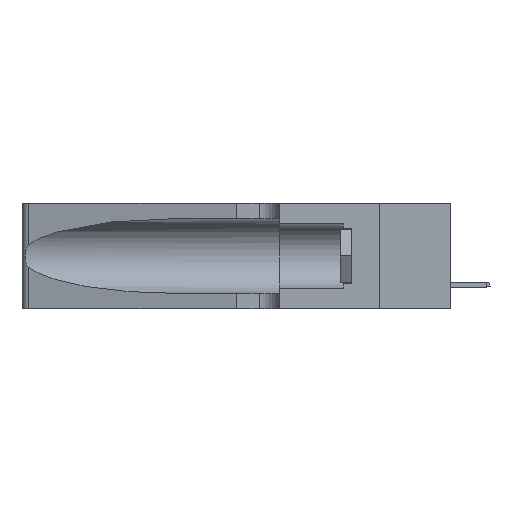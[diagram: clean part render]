
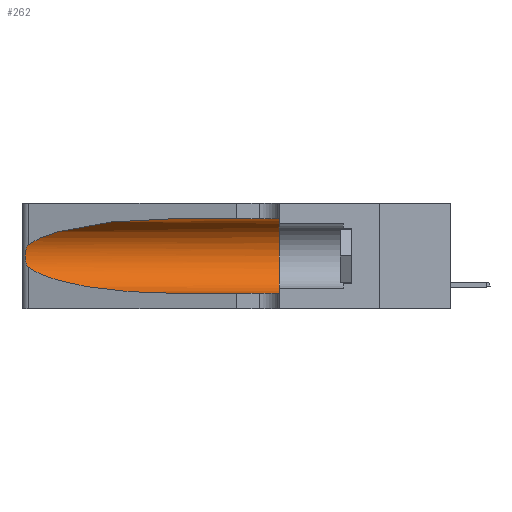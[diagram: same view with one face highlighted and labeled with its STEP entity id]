
A CAD part, left-side view. The second image highlights one B-rep face of the part: STEP entity #262.
In plain terms, the highlighted cylindrical face has radius 3.308 mm (diameter 6.617 mm), a partial arc.
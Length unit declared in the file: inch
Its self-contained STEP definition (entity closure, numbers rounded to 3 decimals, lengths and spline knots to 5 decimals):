
#262 = ADVANCED_FACE ( 'NONE', ( #21001 ), #4156, .F. ) ;
#325 = B_SPLINE_CURVE_WITH_KNOTS ( 'NONE', 3,
 ( #29005, #42861, #22173, #4885, #16473, #26255, #15804, #9646, #16024, #41024, #9871, #19200, #33982, #40575 ),
 .UNSPECIFIED., .F., .F.,
 ( 4, 2, 2, 2, 2, 2, 4 ),
 ( 0., 0.00027, 0.00053, 0.00107, 0.0016, 0.00187, 0.00214 ),
 .UNSPECIFIED. ) ;
#1751 = CIRCLE ( 'NONE', #38068, 0.13025 ) ;
#1962 = EDGE_CURVE ( 'NONE', #35631, #28489, #41548, .T. ) ;
#2505 = AXIS2_PLACEMENT_3D ( 'NONE', #21219, #4380, #3925 ) ;
#2723 = ORIENTED_EDGE ( 'NONE', *, *, #8796, .F. ) ;
#2844 = EDGE_LOOP ( 'NONE', ( #8398, #31038, #37841, #36752, #9120, #2723 ) ) ;
#2851 = CARTESIAN_POINT ( 'NONE',  ( 0.1305, 0.35, 0.31525 ) ) ;
#3925 = DIRECTION ( 'NONE',  ( 0., 0., -1. ) ) ;
#4156 = CYLINDRICAL_SURFACE ( 'NONE', #2505, 0.13025 ) ;
#4380 = DIRECTION ( 'NONE',  ( 0., -1., 0. ) ) ;
#4885 = CARTESIAN_POINT ( 'NONE',  ( 0.25787, 1.23484, 0.2124 ) ) ;
#5344 = CARTESIAN_POINT ( 'NONE',  ( 0.2373, 1.15595, 0.08982 ) ) ;
#5814 =( BOUNDED_CURVE ( )  B_SPLINE_CURVE ( 3, ( #8765, #5344, #39681, #35828 ),
 .UNSPECIFIED., .F., .T. ) 
 B_SPLINE_CURVE_WITH_KNOTS ( ( 4, 4 ),
 ( 3.44316, 4.71239 ),
 .UNSPECIFIED. ) 
 CURVE ( )  GEOMETRIC_REPRESENTATION_ITEM ( )  RATIONAL_B_SPLINE_CURVE ( ( 1., 0.87, 0.87, 1. ) ) 
 REPRESENTATION_ITEM ( '' )  );
#6960 = VERTEX_POINT ( 'NONE', #2851 ) ;
#8398 = ORIENTED_EDGE ( 'NONE', *, *, #1962, .T. ) ;
#8765 = CARTESIAN_POINT ( 'NONE',  ( 0.25487, 1.22718, 0.14631 ) ) ;
#8796 = EDGE_CURVE ( 'NONE', #35631, #6960, #33676, .T. ) ;
#9120 = ORIENTED_EDGE ( 'NONE', *, *, #25398, .F. ) ;
#9646 = CARTESIAN_POINT ( 'NONE',  ( 0.26075, 1.23896, 0.178 ) ) ;
#9871 = CARTESIAN_POINT ( 'NONE',  ( 0.25789, 1.23486, 0.15765 ) ) ;
#10172 = CARTESIAN_POINT ( 'NONE',  ( 0.25487, 1.22718, 0.14631 ) ) ;
#11066 = CARTESIAN_POINT ( 'NONE',  ( 0.2373, 1.15595, 0.28018 ) ) ;
#15804 = CARTESIAN_POINT ( 'NONE',  ( 0.26075, 1.23896, 0.19203 ) ) ;
#16024 = CARTESIAN_POINT ( 'NONE',  ( 0.26017, 1.23833, 0.17102 ) ) ;
#16473 = CARTESIAN_POINT ( 'NONE',  ( 0.25854, 1.2359, 0.20912 ) ) ;
#16642 = CARTESIAN_POINT ( 'NONE',  ( 0.1305, 0.35, 0.05475 ) ) ;
#18571 = CARTESIAN_POINT ( 'NONE',  ( 0.25487, 1.22718, 0.22369 ) ) ;
#19147 = DIRECTION ( 'NONE',  ( 0., 0., 1. ) ) ;
#19200 = CARTESIAN_POINT ( 'NONE',  ( 0.25639, 1.23186, 0.15144 ) ) ;
#21001 = FACE_OUTER_BOUND ( 'NONE', #2844, .T. ) ;
#21219 = CARTESIAN_POINT ( 'NONE',  ( 0.1305, 1.61858, 0.185 ) ) ;
#22173 = CARTESIAN_POINT ( 'NONE',  ( 0.25639, 1.23184, 0.21858 ) ) ;
#22992 = DIRECTION ( 'NONE',  ( 0., -1., 0. ) ) ;
#25398 = EDGE_CURVE ( 'NONE', #6960, #25647, #1751, .T. ) ;
#25619 = CARTESIAN_POINT ( 'NONE',  ( 0.18966, 0.96281, 0.31525 ) ) ;
#25647 = VERTEX_POINT ( 'NONE', #16642 ) ;
#26255 = CARTESIAN_POINT ( 'NONE',  ( 0.26018, 1.23835, 0.19895 ) ) ;
#26322 = LINE ( 'NONE', #34272, #33168 ) ;
#27007 = VERTEX_POINT ( 'NONE', #42317 ) ;
#27752 = EDGE_CURVE ( 'NONE', #27007, #25647, #26322, .T. ) ;
#28489 = VERTEX_POINT ( 'NONE', #35939 ) ;
#28969 = VERTEX_POINT ( 'NONE', #10172 ) ;
#29005 = CARTESIAN_POINT ( 'NONE',  ( 0.25487, 1.22718, 0.22369 ) ) ;
#29395 = CARTESIAN_POINT ( 'NONE',  ( 0.1305, 0.35, 0.185 ) ) ;
#30491 = CARTESIAN_POINT ( 'NONE',  ( 0.1305, 1.61858, 0.31525 ) ) ;
#30800 = VECTOR ( 'NONE', #22992, 39.37008 ) ;
#31038 = ORIENTED_EDGE ( 'NONE', *, *, #34591, .T. ) ;
#32355 = DIRECTION ( 'NONE',  ( 0., 1., 0. ) ) ;
#32754 = CARTESIAN_POINT ( 'NONE',  ( 0.1305, 0.72297, 0.31525 ) ) ;
#33168 = VECTOR ( 'NONE', #40415, 39.37008 ) ;
#33676 = LINE ( 'NONE', #30491, #30800 ) ;
#33982 = CARTESIAN_POINT ( 'NONE',  ( 0.25555, 1.22993, 0.14849 ) ) ;
#34272 = CARTESIAN_POINT ( 'NONE',  ( 0.1305, 1.61858, 0.05475 ) ) ;
#34591 = EDGE_CURVE ( 'NONE', #28489, #28969, #325, .T. ) ;
#35631 = VERTEX_POINT ( 'NONE', #32754 ) ;
#35828 = CARTESIAN_POINT ( 'NONE',  ( 0.1305, 0.72297, 0.05475 ) ) ;
#35939 = CARTESIAN_POINT ( 'NONE',  ( 0.25487, 1.22718, 0.22369 ) ) ;
#36752 = ORIENTED_EDGE ( 'NONE', *, *, #27752, .T. ) ;
#37841 = ORIENTED_EDGE ( 'NONE', *, *, #41416, .T. ) ;
#38068 = AXIS2_PLACEMENT_3D ( 'NONE', #29395, #32355, #19147 ) ;
#39681 = CARTESIAN_POINT ( 'NONE',  ( 0.18966, 0.96281, 0.05475 ) ) ;
#40415 = DIRECTION ( 'NONE',  ( 0., -1., 0. ) ) ;
#40575 = CARTESIAN_POINT ( 'NONE',  ( 0.25487, 1.22718, 0.14631 ) ) ;
#41024 = CARTESIAN_POINT ( 'NONE',  ( 0.25856, 1.23593, 0.16098 ) ) ;
#41394 = CARTESIAN_POINT ( 'NONE',  ( 0.1305, 0.72297, 0.31525 ) ) ;
#41416 = EDGE_CURVE ( 'NONE', #28969, #27007, #5814, .T. ) ;
#41548 =( BOUNDED_CURVE ( )  B_SPLINE_CURVE ( 3, ( #41394, #25619, #11066, #18571 ),
 .UNSPECIFIED., .F., .F. ) 
 B_SPLINE_CURVE_WITH_KNOTS ( ( 4, 4 ),
 ( 1.5708, 2.84003 ),
 .UNSPECIFIED. ) 
 CURVE ( )  GEOMETRIC_REPRESENTATION_ITEM ( )  RATIONAL_B_SPLINE_CURVE ( ( 1., 0.87, 0.87, 1. ) ) 
 REPRESENTATION_ITEM ( '' )  );
#42317 = CARTESIAN_POINT ( 'NONE',  ( 0.1305, 0.72297, 0.05475 ) ) ;
#42861 = CARTESIAN_POINT ( 'NONE',  ( 0.25555, 1.22994, 0.2215 ) ) ;
